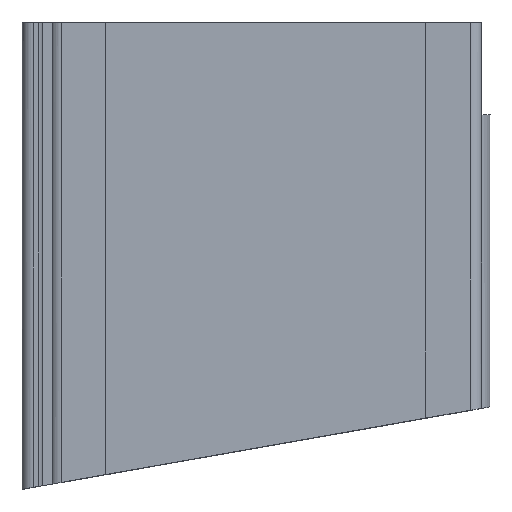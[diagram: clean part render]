
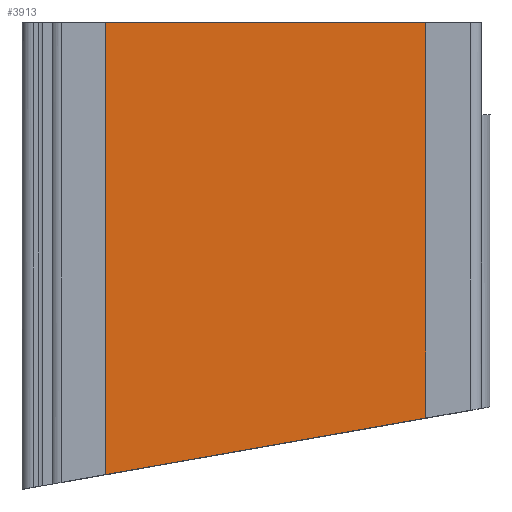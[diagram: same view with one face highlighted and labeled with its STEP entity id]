
A CAD part, top view. The second image highlights one B-rep face of the part: STEP entity #3913.
In plain terms, the highlighted planar face has unit normal (0, 0, 1).
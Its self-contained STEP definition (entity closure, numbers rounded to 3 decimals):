
#32 = PLANE('',#33);
#33 = AXIS2_PLACEMENT_3D('',#34,#35,#36);
#34 = CARTESIAN_POINT('',(-7.567,-47.837,11.849));
#35 = DIRECTION('',(-0.174,0.985,0.));
#36 = DIRECTION('',(-0.985,-0.174,0.));
#854 = VERTEX_POINT('',#855);
#855 = CARTESIAN_POINT('',(-61.925,-57.422,11.622));
#869 = PLANE('',#870);
#870 = AXIS2_PLACEMENT_3D('',#871,#872,#873);
#871 = CARTESIAN_POINT('',(-61.925,6.363,11.405));
#872 = DIRECTION('',(-1.,0.,0.));
#873 = DIRECTION('',(0.,0.,1.));
#881 = EDGE_CURVE('',#854,#882,#884,.T.);
#882 = VERTEX_POINT('',#883);
#883 = CARTESIAN_POINT('',(-16.764,-49.459,11.622));
#884 = SURFACE_CURVE('',#885,(#889,#895),.PCURVE_S1.);
#885 = LINE('',#886,#887);
#886 = CARTESIAN_POINT('',(-29.85,-51.766,11.622));
#887 = VECTOR('',#888,1.);
#888 = DIRECTION('',(0.985,0.174,0.));
#889 = PCURVE('',#32,#890);
#890 = DEFINITIONAL_REPRESENTATION('',(#891),#894);
#891 = B_SPLINE_CURVE_WITH_KNOTS('',1,(#892,#893),.UNSPECIFIED.,.F.,.F.,
  (2,2),(-33.739,14.51),.PIECEWISE_BEZIER_KNOTS.);
#892 = CARTESIAN_POINT('',(56.366,-0.227));
#893 = CARTESIAN_POINT('',(8.118,-0.227));
#894 = ( GEOMETRIC_REPRESENTATION_CONTEXT(2) 
PARAMETRIC_REPRESENTATION_CONTEXT() REPRESENTATION_CONTEXT('2D SPACE',''
  ) );
#895 = PCURVE('',#896,#901);
#896 = PLANE('',#897);
#897 = AXIS2_PLACEMENT_3D('',#898,#899,#900);
#898 = CARTESIAN_POINT('',(-63.077,6.363,11.622));
#899 = DIRECTION('',(0.,0.,1.));
#900 = DIRECTION('',(1.,0.,0.));
#901 = DEFINITIONAL_REPRESENTATION('',(#902),#905);
#902 = B_SPLINE_CURVE_WITH_KNOTS('',1,(#903,#904),.UNSPECIFIED.,.F.,.F.,
  (2,2),(-33.739,14.51),.PIECEWISE_BEZIER_KNOTS.);
#903 = CARTESIAN_POINT('',(0.,-63.987));
#904 = CARTESIAN_POINT('',(47.516,-55.609));
#905 = ( GEOMETRIC_REPRESENTATION_CONTEXT(2) 
PARAMETRIC_REPRESENTATION_CONTEXT() REPRESENTATION_CONTEXT('2D SPACE',''
  ) );
#923 = PLANE('',#924);
#924 = AXIS2_PLACEMENT_3D('',#925,#926,#927);
#925 = CARTESIAN_POINT('',(-16.764,6.363,11.849));
#926 = DIRECTION('',(1.,0.,0.));
#927 = DIRECTION('',(0.,0.,-1.));
#1867 = PLANE('',#1868);
#1868 = AXIS2_PLACEMENT_3D('',#1869,#1870,#1871);
#1869 = CARTESIAN_POINT('',(0.,6.363,-14.288));
#1870 = DIRECTION('',(0.,1.,0.));
#1871 = DIRECTION('',(-1.,0.,0.));
#3771 = EDGE_CURVE('',#854,#3772,#3774,.T.);
#3772 = VERTEX_POINT('',#3773);
#3773 = CARTESIAN_POINT('',(-61.925,6.363,11.622));
#3774 = SURFACE_CURVE('',#3775,(#3779,#3785),.PCURVE_S1.);
#3775 = LINE('',#3776,#3777);
#3776 = CARTESIAN_POINT('',(-61.925,6.363,11.622));
#3777 = VECTOR('',#3778,1.);
#3778 = DIRECTION('',(0.,1.,0.));
#3779 = PCURVE('',#869,#3780);
#3780 = DEFINITIONAL_REPRESENTATION('',(#3781),#3784);
#3781 = B_SPLINE_CURVE_WITH_KNOTS('',1,(#3782,#3783),.UNSPECIFIED.,.F.,
  .F.,(2,2),(-63.784,0.),
  .PIECEWISE_BEZIER_KNOTS.);
#3782 = CARTESIAN_POINT('',(0.217,-63.784));
#3783 = CARTESIAN_POINT('',(0.217,0.));
#3784 = ( GEOMETRIC_REPRESENTATION_CONTEXT(2) 
PARAMETRIC_REPRESENTATION_CONTEXT() REPRESENTATION_CONTEXT('2D SPACE',''
  ) );
#3785 = PCURVE('',#896,#3786);
#3786 = DEFINITIONAL_REPRESENTATION('',(#3787),#3790);
#3787 = B_SPLINE_CURVE_WITH_KNOTS('',1,(#3788,#3789),.UNSPECIFIED.,.F.,
  .F.,(2,2),(-63.784,0.),
  .PIECEWISE_BEZIER_KNOTS.);
#3788 = CARTESIAN_POINT('',(1.151,-63.784));
#3789 = CARTESIAN_POINT('',(1.151,0.));
#3790 = ( GEOMETRIC_REPRESENTATION_CONTEXT(2) 
PARAMETRIC_REPRESENTATION_CONTEXT() REPRESENTATION_CONTEXT('2D SPACE',''
  ) );
#3913 = ADVANCED_FACE('',(#3914),#896,.T.);
#3914 = FACE_BOUND('',#3915,.T.);
#3915 = EDGE_LOOP('',(#3916,#3917,#3918,#3939));
#3916 = ORIENTED_EDGE('',*,*,#3771,.F.);
#3917 = ORIENTED_EDGE('',*,*,#881,.T.);
#3918 = ORIENTED_EDGE('',*,*,#3919,.F.);
#3919 = EDGE_CURVE('',#3920,#882,#3922,.T.);
#3920 = VERTEX_POINT('',#3921);
#3921 = CARTESIAN_POINT('',(-16.764,6.363,11.622));
#3922 = SURFACE_CURVE('',#3923,(#3927,#3933),.PCURVE_S1.);
#3923 = LINE('',#3924,#3925);
#3924 = CARTESIAN_POINT('',(-16.764,6.363,11.622));
#3925 = VECTOR('',#3926,1.);
#3926 = DIRECTION('',(0.,-1.,0.));
#3927 = PCURVE('',#896,#3928);
#3928 = DEFINITIONAL_REPRESENTATION('',(#3929),#3932);
#3929 = B_SPLINE_CURVE_WITH_KNOTS('',1,(#3930,#3931),.UNSPECIFIED.,.F.,
  .F.,(2,2),(0.,55.821),
  .PIECEWISE_BEZIER_KNOTS.);
#3930 = CARTESIAN_POINT('',(46.313,0.));
#3931 = CARTESIAN_POINT('',(46.313,-55.821));
#3932 = ( GEOMETRIC_REPRESENTATION_CONTEXT(2) 
PARAMETRIC_REPRESENTATION_CONTEXT() REPRESENTATION_CONTEXT('2D SPACE',''
  ) );
#3933 = PCURVE('',#923,#3934);
#3934 = DEFINITIONAL_REPRESENTATION('',(#3935),#3938);
#3935 = B_SPLINE_CURVE_WITH_KNOTS('',1,(#3936,#3937),.UNSPECIFIED.,.F.,
  .F.,(2,2),(0.,55.821),
  .PIECEWISE_BEZIER_KNOTS.);
#3936 = CARTESIAN_POINT('',(0.227,0.));
#3937 = CARTESIAN_POINT('',(0.227,-55.821));
#3938 = ( GEOMETRIC_REPRESENTATION_CONTEXT(2) 
PARAMETRIC_REPRESENTATION_CONTEXT() REPRESENTATION_CONTEXT('2D SPACE',''
  ) );
#3939 = ORIENTED_EDGE('',*,*,#3940,.F.);
#3940 = EDGE_CURVE('',#3772,#3920,#3941,.T.);
#3941 = SURFACE_CURVE('',#3942,(#3946,#3953),.PCURVE_S1.);
#3942 = LINE('',#3943,#3944);
#3943 = CARTESIAN_POINT('',(-63.077,6.363,11.622));
#3944 = VECTOR('',#3945,1.);
#3945 = DIRECTION('',(1.,0.,0.));
#3946 = PCURVE('',#896,#3947);
#3947 = DEFINITIONAL_REPRESENTATION('',(#3948),#3952);
#3948 = LINE('',#3949,#3950);
#3949 = CARTESIAN_POINT('',(0.,0.));
#3950 = VECTOR('',#3951,1.);
#3951 = DIRECTION('',(1.,0.));
#3952 = ( GEOMETRIC_REPRESENTATION_CONTEXT(2) 
PARAMETRIC_REPRESENTATION_CONTEXT() REPRESENTATION_CONTEXT('2D SPACE',''
  ) );
#3953 = PCURVE('',#1867,#3954);
#3954 = DEFINITIONAL_REPRESENTATION('',(#3955),#3959);
#3955 = LINE('',#3956,#3957);
#3956 = CARTESIAN_POINT('',(63.077,25.909));
#3957 = VECTOR('',#3958,1.);
#3958 = DIRECTION('',(-1.,0.));
#3959 = ( GEOMETRIC_REPRESENTATION_CONTEXT(2) 
PARAMETRIC_REPRESENTATION_CONTEXT() REPRESENTATION_CONTEXT('2D SPACE',''
  ) );
